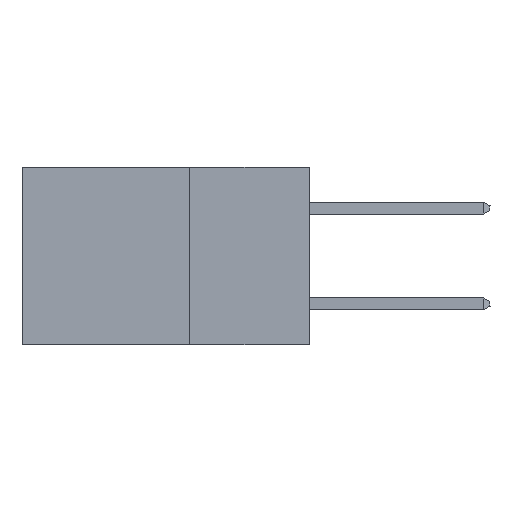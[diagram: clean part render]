
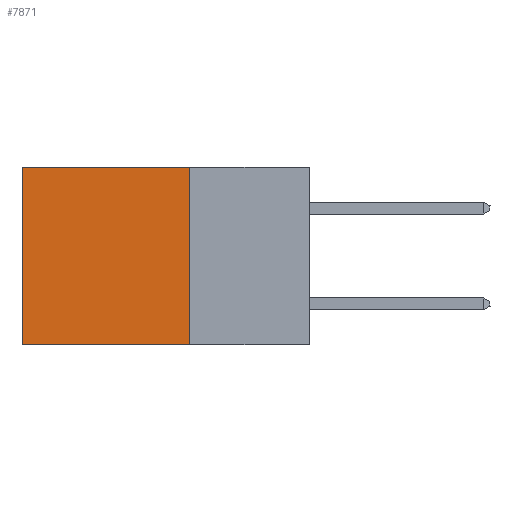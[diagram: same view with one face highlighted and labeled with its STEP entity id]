
A CAD part, left-side view. The second image highlights one B-rep face of the part: STEP entity #7871.
In plain terms, the highlighted planar face has unit normal (-1, 0, 0).
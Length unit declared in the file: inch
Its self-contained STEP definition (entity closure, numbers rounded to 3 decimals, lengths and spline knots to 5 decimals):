
#377 = AXIS2_PLACEMENT_3D ( 'NONE', #9860, #16518, #1016 ) ;
#1016 = DIRECTION ( 'NONE',  ( 0., 0., -1. ) ) ;
#1190 = EDGE_CURVE ( 'NONE', #16298, #5835, #2595, .T. ) ;
#1372 = VECTOR ( 'NONE', #3716, 39.37008 ) ;
#2304 = DIRECTION ( 'NONE',  ( 0., 0., -1. ) ) ;
#2595 = LINE ( 'NONE', #11411, #16314 ) ;
#2865 = CARTESIAN_POINT ( 'NONE',  ( 0.2875, 0.25, -0.37 ) ) ;
#2917 = DIRECTION ( 'NONE',  ( 0., 1., 0. ) ) ;
#3716 = DIRECTION ( 'NONE',  ( 0., 0., -1. ) ) ;
#4377 = VERTEX_POINT ( 'NONE', #13868 ) ;
#4616 = EDGE_CURVE ( 'NONE', #16298, #4377, #13963, .T. ) ;
#4783 = LINE ( 'NONE', #6474, #1372 ) ;
#5798 = ORIENTED_EDGE ( 'NONE', *, *, #7606, .T. ) ;
#5835 = VERTEX_POINT ( 'NONE', #12407 ) ;
#6248 = EDGE_LOOP ( 'NONE', ( #5798, #15877, #14035, #12611 ) ) ;
#6474 = CARTESIAN_POINT ( 'NONE',  ( 0.2875, 0.6, 0. ) ) ;
#7606 = EDGE_CURVE ( 'NONE', #4377, #7798, #4783, .T. ) ;
#7798 = VERTEX_POINT ( 'NONE', #9368 ) ;
#7871 = ADVANCED_FACE ( 'NONE', ( #12219 ), #11285, .F. ) ;
#9368 = CARTESIAN_POINT ( 'NONE',  ( 0.2875, 0.6, -0.37 ) ) ;
#9860 = CARTESIAN_POINT ( 'NONE',  ( 0.2875, 0.25, 0. ) ) ;
#10531 = VECTOR ( 'NONE', #15726, 39.37008 ) ;
#11285 = PLANE ( 'NONE',  #377 ) ;
#11411 = CARTESIAN_POINT ( 'NONE',  ( 0.2875, 0.25, 0. ) ) ;
#12219 = FACE_OUTER_BOUND ( 'NONE', #6248, .T. ) ;
#12407 = CARTESIAN_POINT ( 'NONE',  ( 0.2875, 0.25, -0.37 ) ) ;
#12611 = ORIENTED_EDGE ( 'NONE', *, *, #4616, .T. ) ;
#13296 = CARTESIAN_POINT ( 'NONE',  ( 0.2875, 0.25, 0. ) ) ;
#13868 = CARTESIAN_POINT ( 'NONE',  ( 0.2875, 0.6, 0. ) ) ;
#13963 = LINE ( 'NONE', #13296, #10531 ) ;
#14035 = ORIENTED_EDGE ( 'NONE', *, *, #1190, .F. ) ;
#14183 = EDGE_CURVE ( 'NONE', #5835, #7798, #15189, .T. ) ;
#14900 = CARTESIAN_POINT ( 'NONE',  ( 0.2875, 0.25, 0. ) ) ;
#15189 = LINE ( 'NONE', #2865, #15777 ) ;
#15726 = DIRECTION ( 'NONE',  ( 0., 1., 0. ) ) ;
#15777 = VECTOR ( 'NONE', #2917, 39.37008 ) ;
#15877 = ORIENTED_EDGE ( 'NONE', *, *, #14183, .F. ) ;
#16298 = VERTEX_POINT ( 'NONE', #14900 ) ;
#16314 = VECTOR ( 'NONE', #2304, 39.37008 ) ;
#16518 = DIRECTION ( 'NONE',  ( 1., 0., 0. ) ) ;
